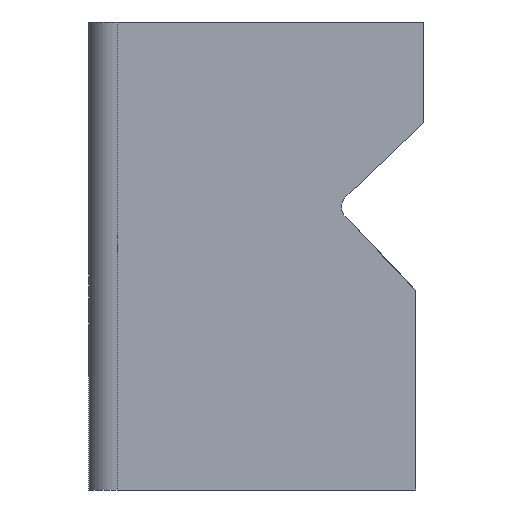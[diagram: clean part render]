
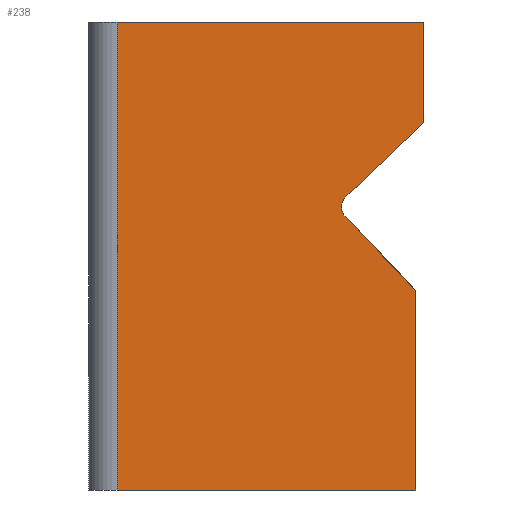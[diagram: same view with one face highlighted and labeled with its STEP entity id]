
A CAD part, front view. The second image highlights one B-rep face of the part: STEP entity #238.
In plain terms, the highlighted planar face has unit normal (0, -1, 0).
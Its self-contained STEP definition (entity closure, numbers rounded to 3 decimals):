
#2 = AXIS2_PLACEMENT_3D ( 'NONE', #447, #551, #161 ) ;
#5 = CARTESIAN_POINT ( 'NONE',  ( -10.73, 0., 0. ) ) ;
#8 = CARTESIAN_POINT ( 'NONE',  ( -2.712, 0., -6.12 ) ) ;
#18 = VERTEX_POINT ( 'NONE', #375 ) ;
#19 = EDGE_CURVE ( 'NONE', #140, #18, #368, .T. ) ;
#30 = EDGE_LOOP ( 'NONE', ( #280, #190, #296, #329, #408, #527, #518, #40 ) ) ;
#37 = DIRECTION ( 'NONE',  ( 0.691, 0., -0.723 ) ) ;
#40 = ORIENTED_EDGE ( 'NONE', *, *, #625, .F. ) ;
#57 = FACE_OUTER_BOUND ( 'NONE', #30, .T. ) ;
#64 = AXIS2_PLACEMENT_3D ( 'NONE', #106, #502, #258 ) ;
#84 = CARTESIAN_POINT ( 'NONE',  ( -10.73, 0., -16.4 ) ) ;
#87 = LINE ( 'NONE', #378, #216 ) ;
#94 = VECTOR ( 'NONE', #285, 1000. ) ;
#97 = CARTESIAN_POINT ( 'NONE',  ( -0.27, 0., -16.4 ) ) ;
#99 = LINE ( 'NONE', #415, #598 ) ;
#102 = LINE ( 'NONE', #451, #529 ) ;
#106 = CARTESIAN_POINT ( 'NONE',  ( -2.366, 0., -6.481 ) ) ;
#116 = VERTEX_POINT ( 'NONE', #298 ) ;
#134 = VECTOR ( 'NONE', #192, 1000. ) ;
#140 = VERTEX_POINT ( 'NONE', #5 ) ;
#143 = VERTEX_POINT ( 'NONE', #8 ) ;
#146 = CIRCLE ( 'NONE', #2, 0.5 ) ;
#161 = DIRECTION ( 'NONE',  ( 0., 0., -1. ) ) ;
#172 = EDGE_CURVE ( 'NONE', #610, #506, #102, .T. ) ;
#186 = CARTESIAN_POINT ( 'NONE',  ( -11.73, 0., 0. ) ) ;
#190 = ORIENTED_EDGE ( 'NONE', *, *, #438, .T. ) ;
#192 = DIRECTION ( 'NONE',  ( 1., 0., 0. ) ) ;
#202 = CARTESIAN_POINT ( 'NONE',  ( 0., 0., 0. ) ) ;
#216 = VECTOR ( 'NONE', #631, 1000. ) ;
#238 = ADVANCED_FACE ( 'NONE', ( #57 ), #545, .T. ) ;
#258 = DIRECTION ( 'NONE',  ( 0., 0., -1. ) ) ;
#274 = CARTESIAN_POINT ( 'NONE',  ( -10.73, 0., -16.4 ) ) ;
#280 = ORIENTED_EDGE ( 'NONE', *, *, #19, .F. ) ;
#281 = CARTESIAN_POINT ( 'NONE',  ( -2.728, 0., -6.827 ) ) ;
#285 = DIRECTION ( 'NONE',  ( 0., 0., -1. ) ) ;
#296 = ORIENTED_EDGE ( 'NONE', *, *, #172, .F. ) ;
#298 = CARTESIAN_POINT ( 'NONE',  ( 0., 0., -3.53 ) ) ;
#329 = ORIENTED_EDGE ( 'NONE', *, *, #487, .F. ) ;
#368 = LINE ( 'NONE', #186, #134 ) ;
#370 = CARTESIAN_POINT ( 'NONE',  ( -0.27, 0., -9.4 ) ) ;
#373 = EDGE_CURVE ( 'NONE', #143, #458, #146, .T. ) ;
#375 = CARTESIAN_POINT ( 'NONE',  ( 0., 0., 0. ) ) ;
#378 = CARTESIAN_POINT ( 'NONE',  ( 0., 0., -3.53 ) ) ;
#396 = DIRECTION ( 'NONE',  ( -1., 0., 0. ) ) ;
#399 = EDGE_CURVE ( 'NONE', #458, #525, #99, .T. ) ;
#408 = ORIENTED_EDGE ( 'NONE', *, *, #399, .F. ) ;
#415 = CARTESIAN_POINT ( 'NONE',  ( -2.728, 0., -6.827 ) ) ;
#420 = LINE ( 'NONE', #370, #588 ) ;
#438 = EDGE_CURVE ( 'NONE', #140, #506, #566, .T. ) ;
#447 = CARTESIAN_POINT ( 'NONE',  ( -2.366, 0., -6.481 ) ) ;
#451 = CARTESIAN_POINT ( 'NONE',  ( -0.27, 0., -16.4 ) ) ;
#458 = VERTEX_POINT ( 'NONE', #281 ) ;
#487 = EDGE_CURVE ( 'NONE', #525, #610, #420, .T. ) ;
#496 = CARTESIAN_POINT ( 'NONE',  ( -0.27, 0., -9.4 ) ) ;
#502 = DIRECTION ( 'NONE',  ( 0., -1., 0. ) ) ;
#506 = VERTEX_POINT ( 'NONE', #84 ) ;
#511 = EDGE_CURVE ( 'NONE', #116, #143, #87, .T. ) ;
#518 = ORIENTED_EDGE ( 'NONE', *, *, #511, .F. ) ;
#525 = VERTEX_POINT ( 'NONE', #496 ) ;
#527 = ORIENTED_EDGE ( 'NONE', *, *, #373, .F. ) ;
#529 = VECTOR ( 'NONE', #396, 1000. ) ;
#530 = LINE ( 'NONE', #202, #94 ) ;
#545 = PLANE ( 'NONE',  #64 ) ;
#551 = DIRECTION ( 'NONE',  ( 0., -1., 0. ) ) ;
#562 = DIRECTION ( 'NONE',  ( 0., 0., -1. ) ) ;
#566 = LINE ( 'NONE', #274, #616 ) ;
#588 = VECTOR ( 'NONE', #618, 1000. ) ;
#598 = VECTOR ( 'NONE', #37, 1000. ) ;
#610 = VERTEX_POINT ( 'NONE', #97 ) ;
#616 = VECTOR ( 'NONE', #562, 1000. ) ;
#618 = DIRECTION ( 'NONE',  ( 0., 0., -1. ) ) ;
#625 = EDGE_CURVE ( 'NONE', #18, #116, #530, .T. ) ;
#631 = DIRECTION ( 'NONE',  ( -0.723, 0., -0.691 ) ) ;
